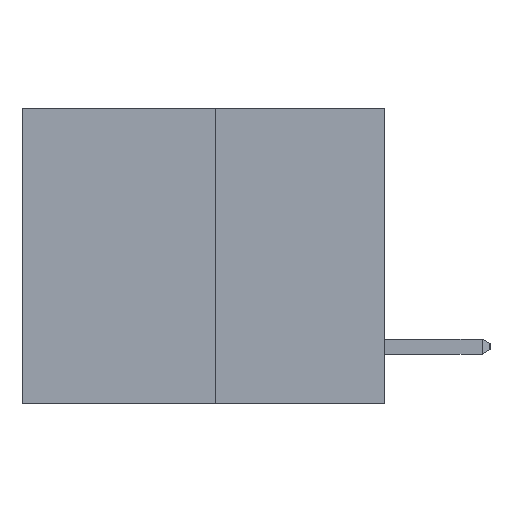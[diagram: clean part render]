
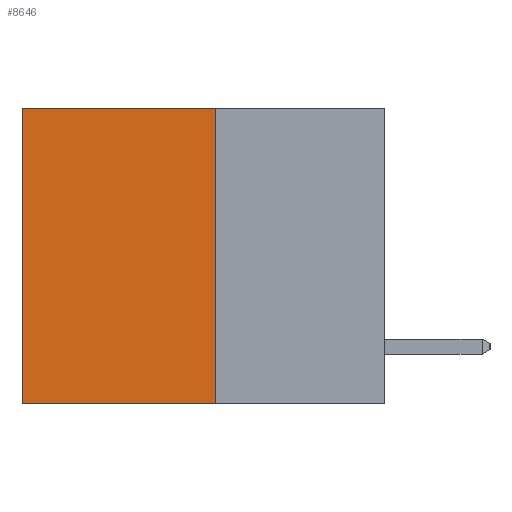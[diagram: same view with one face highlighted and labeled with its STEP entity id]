
A CAD part, left-side view. The second image highlights one B-rep face of the part: STEP entity #8646.
In plain terms, the highlighted planar face has unit normal (-1, 0, 0).
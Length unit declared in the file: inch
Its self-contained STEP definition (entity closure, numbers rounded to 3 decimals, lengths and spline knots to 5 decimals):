
#201 = LINE ( 'NONE', #2462, #3849 ) ;
#498 = DIRECTION ( 'NONE',  ( 0., 1., 0. ) ) ;
#528 = ORIENTED_EDGE ( 'NONE', *, *, #7268, .F. ) ;
#1059 = VERTEX_POINT ( 'NONE', #2530 ) ;
#1067 = EDGE_CURVE ( 'NONE', #1932, #1059, #201, .T. ) ;
#1323 = ORIENTED_EDGE ( 'NONE', *, *, #1067, .F. ) ;
#1932 = VERTEX_POINT ( 'NONE', #2342 ) ;
#2094 = VERTEX_POINT ( 'NONE', #7668 ) ;
#2212 = DIRECTION ( 'NONE',  ( 0., 0., -1. ) ) ;
#2258 = EDGE_CURVE ( 'NONE', #2094, #2589, #7180, .T. ) ;
#2342 = CARTESIAN_POINT ( 'NONE',  ( 0.3165, 0.28, -0.49 ) ) ;
#2462 = CARTESIAN_POINT ( 'NONE',  ( 0.3165, 0.28, -0.49 ) ) ;
#2530 = CARTESIAN_POINT ( 'NONE',  ( 0.3165, 0.6, -0.49 ) ) ;
#2589 = VERTEX_POINT ( 'NONE', #7532 ) ;
#2799 = CARTESIAN_POINT ( 'NONE',  ( 0.3165, 0.6, -0.49 ) ) ;
#2922 = ORIENTED_EDGE ( 'NONE', *, *, #9682, .T. ) ;
#3004 = CARTESIAN_POINT ( 'NONE',  ( 0.3165, 0.28, 0. ) ) ;
#3294 = VECTOR ( 'NONE', #498, 39.37008 ) ;
#3341 = CARTESIAN_POINT ( 'NONE',  ( 0.3165, 0.28, -0.49 ) ) ;
#3849 = VECTOR ( 'NONE', #9219, 39.37008 ) ;
#3863 = CARTESIAN_POINT ( 'NONE',  ( 0.3165, 0.28, -0.49 ) ) ;
#3952 = EDGE_LOOP ( 'NONE', ( #2922, #1323, #528, #4374 ) ) ;
#4374 = ORIENTED_EDGE ( 'NONE', *, *, #2258, .T. ) ;
#4615 = VECTOR ( 'NONE', #9151, 39.37008 ) ;
#5234 = DIRECTION ( 'NONE',  ( 0., 0., -1. ) ) ;
#5403 = DIRECTION ( 'NONE',  ( 1., 0., 0. ) ) ;
#6287 = AXIS2_PLACEMENT_3D ( 'NONE', #3863, #5403, #2212 ) ;
#6508 = FACE_OUTER_BOUND ( 'NONE', #3952, .T. ) ;
#6538 = LINE ( 'NONE', #3341, #4615 ) ;
#7000 = LINE ( 'NONE', #2799, #8966 ) ;
#7180 = LINE ( 'NONE', #3004, #3294 ) ;
#7268 = EDGE_CURVE ( 'NONE', #2094, #1932, #6538, .T. ) ;
#7532 = CARTESIAN_POINT ( 'NONE',  ( 0.3165, 0.6, 0. ) ) ;
#7668 = CARTESIAN_POINT ( 'NONE',  ( 0.3165, 0.28, 0. ) ) ;
#8646 = ADVANCED_FACE ( 'NONE', ( #6508 ), #10430, .F. ) ;
#8966 = VECTOR ( 'NONE', #5234, 39.37008 ) ;
#9151 = DIRECTION ( 'NONE',  ( 0., 0., -1. ) ) ;
#9219 = DIRECTION ( 'NONE',  ( 0., 1., 0. ) ) ;
#9682 = EDGE_CURVE ( 'NONE', #2589, #1059, #7000, .T. ) ;
#10430 = PLANE ( 'NONE',  #6287 ) ;
